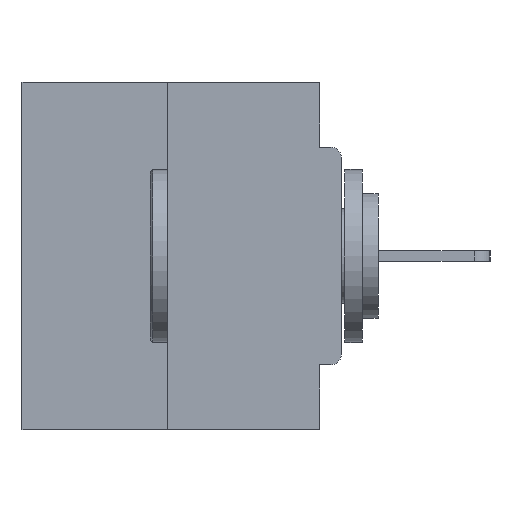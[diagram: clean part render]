
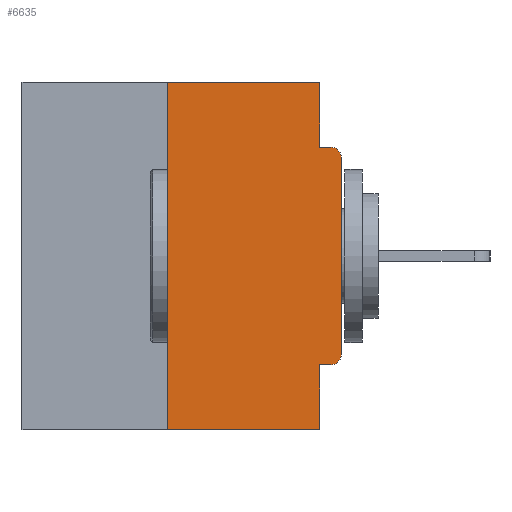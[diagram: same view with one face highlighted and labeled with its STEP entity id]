
A CAD part, left-side view. The second image highlights one B-rep face of the part: STEP entity #6635.
In plain terms, the highlighted planar face has unit normal (-1, 0, 0).
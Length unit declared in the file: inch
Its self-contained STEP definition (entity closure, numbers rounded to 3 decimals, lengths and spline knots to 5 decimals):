
#307 = VERTEX_POINT ( 'NONE', #32277 ) ;
#518 = CARTESIAN_POINT ( 'NONE',  ( 0., 0.031, -0.5 ) ) ;
#1423 = CARTESIAN_POINT ( 'NONE',  ( 0., 0.46, 0. ) ) ;
#2359 = CARTESIAN_POINT ( 'NONE',  ( 0., 0.031, -0.4065 ) ) ;
#2809 = EDGE_CURVE ( 'NONE', #21194, #13832, #28252, .T. ) ;
#2867 = DIRECTION ( 'NONE',  ( 0., 0., -1. ) ) ;
#3177 = VECTOR ( 'NONE', #13929, 39.37008 ) ;
#3330 = EDGE_CURVE ( 'NONE', #18449, #8782, #13044, .T. ) ;
#3353 = DIRECTION ( 'NONE',  ( -1., 0., 0. ) ) ;
#4392 = DIRECTION ( 'NONE',  ( 0., 0., -1. ) ) ;
#4493 = CARTESIAN_POINT ( 'NONE',  ( 0., 0.015, -0.0935 ) ) ;
#4952 = VECTOR ( 'NONE', #12190, 39.37008 ) ;
#5484 = EDGE_CURVE ( 'NONE', #5799, #21194, #25191, .T. ) ;
#5500 = ORIENTED_EDGE ( 'NONE', *, *, #10099, .F. ) ;
#5584 = CARTESIAN_POINT ( 'NONE',  ( 0., 0., 0. ) ) ;
#5656 = CARTESIAN_POINT ( 'NONE',  ( 0., 0.25, 0. ) ) ;
#5799 = VERTEX_POINT ( 'NONE', #14696 ) ;
#6445 = LINE ( 'NONE', #9610, #19139 ) ;
#6635 = ADVANCED_FACE ( 'NONE', ( #10243 ), #20394, .F. ) ;
#6693 = VECTOR ( 'NONE', #4392, 39.37008 ) ;
#7092 = VECTOR ( 'NONE', #23583, 39.37008 ) ;
#8782 = VERTEX_POINT ( 'NONE', #28461 ) ;
#9541 = VERTEX_POINT ( 'NONE', #16211 ) ;
#9610 = CARTESIAN_POINT ( 'NONE',  ( 0., 0., -0.0935 ) ) ;
#10002 = ORIENTED_EDGE ( 'NONE', *, *, #2809, .T. ) ;
#10099 = EDGE_CURVE ( 'NONE', #307, #28558, #6445, .T. ) ;
#10182 = EDGE_CURVE ( 'NONE', #9541, #8782, #32439, .T. ) ;
#10243 = FACE_OUTER_BOUND ( 'NONE', #24472, .T. ) ;
#10529 = AXIS2_PLACEMENT_3D ( 'NONE', #17245, #27414, #13375 ) ;
#11068 = CARTESIAN_POINT ( 'NONE',  ( 0., 0., -0.1085 ) ) ;
#11489 = VECTOR ( 'NONE', #23662, 39.37008 ) ;
#12190 = DIRECTION ( 'NONE',  ( 0., 1., 0. ) ) ;
#13044 = LINE ( 'NONE', #518, #25239 ) ;
#13339 = ORIENTED_EDGE ( 'NONE', *, *, #17806, .F. ) ;
#13375 = DIRECTION ( 'NONE',  ( 0., 0., -1. ) ) ;
#13768 = LINE ( 'NONE', #1423, #3177 ) ;
#13832 = VERTEX_POINT ( 'NONE', #11068 ) ;
#13929 = DIRECTION ( 'NONE',  ( 0., -1., 0. ) ) ;
#14055 = ORIENTED_EDGE ( 'NONE', *, *, #27892, .F. ) ;
#14469 = AXIS2_PLACEMENT_3D ( 'NONE', #30224, #22733, #14717 ) ;
#14691 = LINE ( 'NONE', #32035, #4952 ) ;
#14696 = CARTESIAN_POINT ( 'NONE',  ( 0., 0.015, -0.4065 ) ) ;
#14717 = DIRECTION ( 'NONE',  ( 0., 0., -1. ) ) ;
#15488 = LINE ( 'NONE', #5656, #11489 ) ;
#16211 = CARTESIAN_POINT ( 'NONE',  ( 0., 0.25, -0.5 ) ) ;
#16800 = DIRECTION ( 'NONE',  ( 0., -1., 0. ) ) ;
#17073 = CARTESIAN_POINT ( 'NONE',  ( 0., 0.031, 0. ) ) ;
#17245 = CARTESIAN_POINT ( 'NONE',  ( 0., 0.46, 0. ) ) ;
#17806 = EDGE_CURVE ( 'NONE', #17950, #23174, #13768, .T. ) ;
#17950 = VERTEX_POINT ( 'NONE', #22769 ) ;
#18449 = VERTEX_POINT ( 'NONE', #2359 ) ;
#19139 = VECTOR ( 'NONE', #16800, 39.37008 ) ;
#19228 = ORIENTED_EDGE ( 'NONE', *, *, #10182, .T. ) ;
#19476 = EDGE_CURVE ( 'NONE', #13832, #28558, #28847, .T. ) ;
#20394 = PLANE ( 'NONE',  #10529 ) ;
#21194 = VERTEX_POINT ( 'NONE', #21574 ) ;
#21467 = AXIS2_PLACEMENT_3D ( 'NONE', #25541, #3353, #2867 ) ;
#21574 = CARTESIAN_POINT ( 'NONE',  ( 0., 0., -0.3915 ) ) ;
#22336 = VECTOR ( 'NONE', #32127, 39.37008 ) ;
#22733 = DIRECTION ( 'NONE',  ( -1., 0., 0. ) ) ;
#22769 = CARTESIAN_POINT ( 'NONE',  ( 0., 0.25, 0. ) ) ;
#22958 = ORIENTED_EDGE ( 'NONE', *, *, #23006, .F. ) ;
#23006 = EDGE_CURVE ( 'NONE', #9541, #17950, #15488, .T. ) ;
#23174 = VERTEX_POINT ( 'NONE', #23994 ) ;
#23230 = DIRECTION ( 'NONE',  ( 0., 0., -1. ) ) ;
#23389 = ORIENTED_EDGE ( 'NONE', *, *, #25213, .F. ) ;
#23583 = DIRECTION ( 'NONE',  ( 0., 0., 1. ) ) ;
#23662 = DIRECTION ( 'NONE',  ( 0., 0., 1. ) ) ;
#23994 = CARTESIAN_POINT ( 'NONE',  ( 0., 0.031, 0. ) ) ;
#24472 = EDGE_LOOP ( 'NONE', ( #13339, #22958, #19228, #29911, #23389, #24905, #10002, #28601, #5500, #14055 ) ) ;
#24905 = ORIENTED_EDGE ( 'NONE', *, *, #5484, .T. ) ;
#25191 = CIRCLE ( 'NONE', #21467, 0.015 ) ;
#25213 = EDGE_CURVE ( 'NONE', #5799, #18449, #14691, .T. ) ;
#25239 = VECTOR ( 'NONE', #23230, 39.37008 ) ;
#25541 = CARTESIAN_POINT ( 'NONE',  ( 0., 0.015, -0.3915 ) ) ;
#26956 = CARTESIAN_POINT ( 'NONE',  ( 0., 0.46, -0.5 ) ) ;
#27414 = DIRECTION ( 'NONE',  ( 1., 0., 0. ) ) ;
#27892 = EDGE_CURVE ( 'NONE', #23174, #307, #29588, .T. ) ;
#28252 = LINE ( 'NONE', #5584, #7092 ) ;
#28461 = CARTESIAN_POINT ( 'NONE',  ( 0., 0.031, -0.5 ) ) ;
#28558 = VERTEX_POINT ( 'NONE', #4493 ) ;
#28601 = ORIENTED_EDGE ( 'NONE', *, *, #19476, .T. ) ;
#28847 = CIRCLE ( 'NONE', #14469, 0.015 ) ;
#29588 = LINE ( 'NONE', #17073, #6693 ) ;
#29911 = ORIENTED_EDGE ( 'NONE', *, *, #3330, .F. ) ;
#30224 = CARTESIAN_POINT ( 'NONE',  ( 0., 0.015, -0.1085 ) ) ;
#32035 = CARTESIAN_POINT ( 'NONE',  ( 0., 0., -0.4065 ) ) ;
#32127 = DIRECTION ( 'NONE',  ( 0., -1., 0. ) ) ;
#32277 = CARTESIAN_POINT ( 'NONE',  ( 0., 0.031, -0.0935 ) ) ;
#32439 = LINE ( 'NONE', #26956, #22336 ) ;
